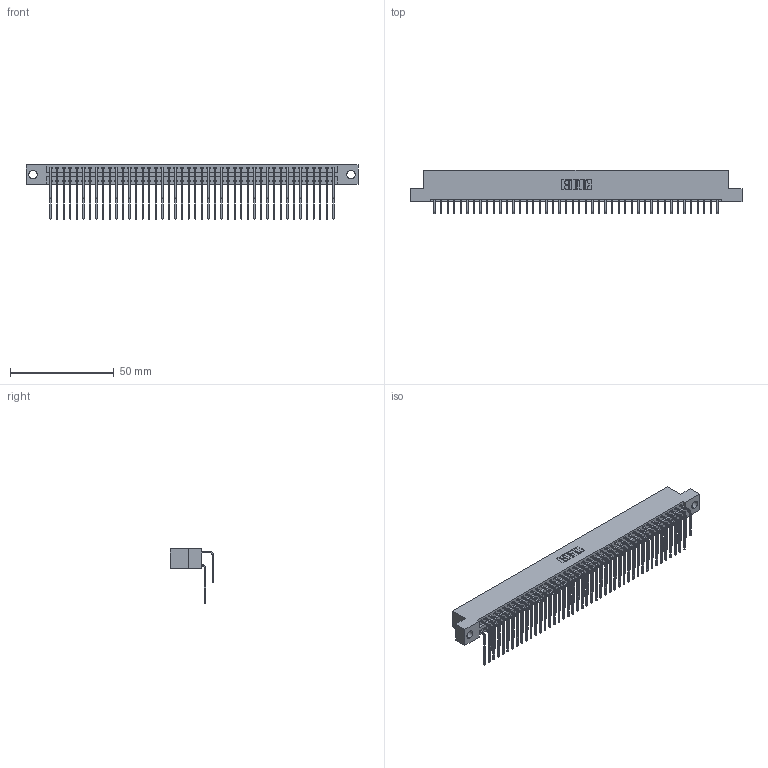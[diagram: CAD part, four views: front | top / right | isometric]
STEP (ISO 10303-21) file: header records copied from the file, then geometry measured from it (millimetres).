
FILE_DESCRIPTION (( 'STEP AP203' ), '1' );
FILE_NAME ('346-088-559-204.STEP', '2022-05-26T02:18:25', ( '' ), ( '' ), 'SwSTEP 2.0', 'SolidWorks 2020', '' );
FILE_SCHEMA (( 'CONFIG_CONTROL_DESIGN' ));
Length unit declared in the file: inch
Products named in the file (4): 345-292-001_559 Tail - 2; 346 Part_Flush Mounting Lugs - 0.156 Dia-TH; 346-088-559-204; 345-292-001_558 559 Tail - 1
Assembly tree (89 placements, depth 2):
  346-088-559-204
    346 Part_Flush Mounting Lugs - 0.156 Dia-TH
    345-292-001_558 559 Tail - 1  x44
    345-292-001_559 Tail - 2  x44
Bounding box: 160.27 x 20.89 x 26.16 mm (x, y, z)
Volume: 16045.9 mm3; surface area: 24370.9 mm2
Topology: 89 solids, 89 shells, 4888 faces, 14533 edges, 9570 vertices
Faces by surface type: plane 3346, cylinder 1542
Entity records: 30649 total; most frequent: CARTESIAN_POINT 5105, ORIENTED_EDGE 4986, DIRECTION 4521, EDGE_CURVE 2493, VECTOR 2145, LINE 2145, VERTEX_POINT 1658, AXIS2_PLACEMENT_3D 1188
